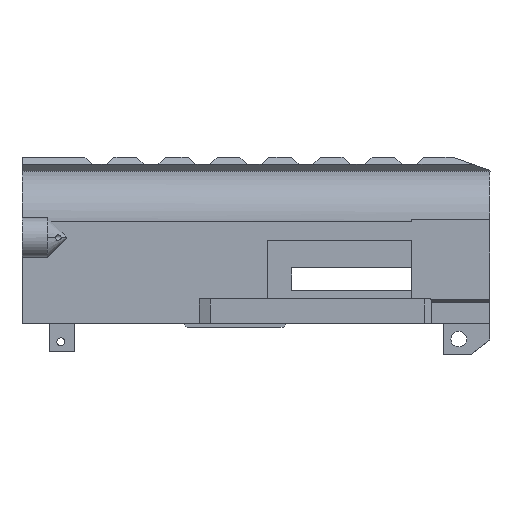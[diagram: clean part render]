
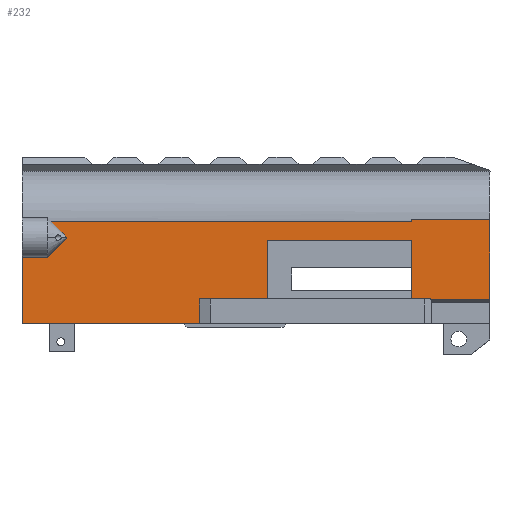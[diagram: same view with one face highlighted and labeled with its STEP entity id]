
A CAD part, top view. The second image highlights one B-rep face of the part: STEP entity #232.
In plain terms, the highlighted planar face has unit normal (0, 0, 1).
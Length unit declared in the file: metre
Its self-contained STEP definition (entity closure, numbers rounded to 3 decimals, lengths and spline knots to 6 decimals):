
#232=ADVANCED_FACE('5:5640',(#699),#700,.T.);
#699=FACE_OUTER_BOUND('',#1312,.T.);
#700=PLANE('',#1313);
#1312=EDGE_LOOP('',(#3033,#3034,#3035,#3036,#3037,#3038,#3039,#3040,#3041,#3042,#3043,#3044,#3045,#3046,#3047,#3048,#3049,#3050));
#1313=AXIS2_PLACEMENT_3D('',#3051,#3052,#3053);
#3033=ORIENTED_EDGE('',*,*,#4156,.T.);
#3034=ORIENTED_EDGE('',*,*,#4449,.T.);
#3035=ORIENTED_EDGE('',*,*,#4154,.F.);
#3036=ORIENTED_EDGE('',*,*,#4429,.F.);
#3037=ORIENTED_EDGE('',*,*,#4450,.T.);
#3038=ORIENTED_EDGE('',*,*,#4401,.F.);
#3039=ORIENTED_EDGE('',*,*,#4002,.F.);
#3040=ORIENTED_EDGE('',*,*,#4430,.F.);
#3041=ORIENTED_EDGE('',*,*,#4140,.T.);
#3042=ORIENTED_EDGE('',*,*,#4122,.F.);
#3043=ORIENTED_EDGE('',*,*,#4451,.T.);
#3044=ORIENTED_EDGE('',*,*,#4118,.F.);
#3045=ORIENTED_EDGE('',*,*,#4117,.F.);
#3046=ORIENTED_EDGE('',*,*,#4116,.T.);
#3047=ORIENTED_EDGE('',*,*,#3915,.T.);
#3048=ORIENTED_EDGE('',*,*,#4452,.T.);
#3049=ORIENTED_EDGE('',*,*,#4399,.F.);
#3050=ORIENTED_EDGE('',*,*,#4395,.T.);
#3051=CARTESIAN_POINT('',(-0.001544,-0.005067,0.0201));
#3052=DIRECTION('',(0.0,0.,1.0));
#3053=DIRECTION('',(-1.0,0.0,0.0));
#3915=EDGE_CURVE('5:7011',#4785,#4783,#4786,.T.);
#4002=EDGE_CURVE('5:6045',#4935,#4937,#4938,.T.);
#4116=EDGE_CURVE('5:7008',#5139,#4785,#5140,.T.);
#4117=EDGE_CURVE('5:7005',#5139,#5141,#5142,.T.);
#4118=EDGE_CURVE('5:7002',#5141,#5143,#5144,.T.);
#4122=EDGE_CURVE('5:6999',#5149,#5151,#5152,.T.);
#4140=EDGE_CURVE('5:6996',#5178,#5151,#5179,.T.);
#4154=EDGE_CURVE('5:6984',#5200,#5198,#5202,.T.);
#4156=EDGE_CURVE('5:6981',#5206,#5204,#5207,.T.);
#4395=EDGE_CURVE('5:7017',#5586,#5206,#5587,.T.);
#4399=EDGE_CURVE('5:7014',#5586,#5592,#5593,.T.);
#4401=EDGE_CURVE('5:6990',#4937,#5595,#5596,.T.);
#4429=EDGE_CURVE('5:6987',#5628,#5200,#5630,.T.);
#4430=EDGE_CURVE('5:6993',#5178,#4935,#5631,.T.);
#4449=EDGE_CURVE('5:6291',#5204,#5198,#5657,.T.);
#4450=EDGE_CURVE('5:6492',#5628,#5595,#5658,.T.);
#4451=EDGE_CURVE('5:6204',#5149,#5143,#5659,.T.);
#4452=EDGE_CURVE('5:6504',#4783,#5592,#5660,.T.);
#4783=VERTEX_POINT('',#6201);
#4785=VERTEX_POINT('',#6203);
#4786=LINE('',#6204,#6205);
#4935=VERTEX_POINT('',#6596);
#4937=VERTEX_POINT('',#6599);
#4938=LINE('',#6600,#6601);
#5139=VERTEX_POINT('',#6893);
#5140=LINE('',#6894,#6895);
#5141=VERTEX_POINT('',#6896);
#5142=CIRCLE('',#6897,0.0201);
#5143=VERTEX_POINT('',#6898);
#5144=LINE('',#6899,#6900);
#5149=VERTEX_POINT('',#6906);
#5151=VERTEX_POINT('',#6908);
#5152=LINE('',#6909,#6910);
#5178=VERTEX_POINT('',#6954);
#5179=LINE('',#6955,#6956);
#5198=VERTEX_POINT('',#6986);
#5200=VERTEX_POINT('',#6989);
#5202=LINE('',#6992,#6993);
#5204=VERTEX_POINT('',#6995);
#5206=VERTEX_POINT('',#6998);
#5207=LINE('',#6999,#7000);
#5586=VERTEX_POINT('',#7599);
#5587=LINE('',#7600,#7601);
#5592=VERTEX_POINT('',#7621);
#5593=LINE('',#7622,#7623);
#5595=VERTEX_POINT('',#7625);
#5596=LINE('',#7626,#7627);
#5628=VERTEX_POINT('',#7679);
#5630=LINE('',#7682,#7683);
#5631=LINE('',#7684,#7685);
#5657=LINE('',#7751,#7752);
#5658=LINE('',#7753,#7754);
#5659=LINE('',#7755,#7756);
#5660=LINE('',#7757,#7758);
#6201=CARTESIAN_POINT('',(-0.159682,0.0415,0.0201));
#6203=CARTESIAN_POINT('',(-0.166095,0.047913,0.0201));
#6204=CARTESIAN_POINT('',(-0.159482,0.0413,0.0201));
#6205=VECTOR('',#8150,0.009069);
#6596=CARTESIAN_POINT('',(-0.019032,0.016363,0.0201));
#6599=CARTESIAN_POINT('',(-0.019032,0.039948,0.0201));
#6600=CARTESIAN_POINT('',(-0.019032,0.017441,0.0201));
#6601=VECTOR('',#8292,0.023586);
#6893=CARTESIAN_POINT('',(-0.01905,0.047913,0.0201));
#6894=CARTESIAN_POINT('',(-0.01905,0.047913,0.0201));
#6895=VECTOR('',#8450,0.147045);
#6896=CARTESIAN_POINT('',(-0.01905,0.048502,0.020096));
#6897=AXIS2_PLACEMENT_3D('',#8451,#8452,#8453);
#6898=CARTESIAN_POINT('',(0.0127,0.048502,0.020096));
#6899=CARTESIAN_POINT('',(-0.19405,0.048472,0.020092));
#6900=VECTOR('',#8454,0.03175);
#6906=CARTESIAN_POINT('',(0.0127,0.016229,0.0201));
#6908=CARTESIAN_POINT('',(-0.011605,0.016229,0.0201));
#6909=CARTESIAN_POINT('',(-0.01905,0.016229,0.0201));
#6910=VECTOR('',#8462,0.024305);
#6954=CARTESIAN_POINT('',(-0.011605,0.016363,0.0201));
#6955=CARTESIAN_POINT('',(-0.011605,0.005648,0.0201));
#6956=VECTOR('',#8490,0.000134);
#6986=CARTESIAN_POINT('',(-0.105565,0.006363,0.0201));
#6989=CARTESIAN_POINT('',(-0.105565,0.016363,0.0201));
#6992=CARTESIAN_POINT('',(-0.105565,0.000648,0.0201));
#6993=VECTOR('',#8504,0.000134);
#6995=CARTESIAN_POINT('',(-0.177682,0.006363,0.0201));
#6998=CARTESIAN_POINT('',(-0.177682,0.0333,0.0201));
#6999=CARTESIAN_POINT('',(-0.177682,0.012778,0.0201));
#7000=VECTOR('',#8506,0.001627);
#7599=CARTESIAN_POINT('',(-0.167482,0.0333,0.0201));
#7600=CARTESIAN_POINT('',(-0.167682,0.0333,0.0201));
#7601=VECTOR('',#8808,0.0102);
#7621=CARTESIAN_POINT('',(-0.159682,0.0411,0.0201));
#7622=CARTESIAN_POINT('',(-0.159482,0.0413,0.0201));
#7623=VECTOR('',#8812,0.011031);
#7625=CARTESIAN_POINT('',(-0.078,0.039948,0.0201));
#7626=CARTESIAN_POINT('',(-0.039772,0.039948,0.0201));
#7627=VECTOR('',#8816,0.000018);
#7679=CARTESIAN_POINT('',(-0.078,0.016363,0.0201));
#7682=CARTESIAN_POINT('',(-0.053554,0.016363,0.0201));
#7683=VECTOR('',#8868,0.027565);
#7684=CARTESIAN_POINT('',(-0.053554,0.016363,0.0201));
#7685=VECTOR('',#8869,0.007427);
#7751=CARTESIAN_POINT('',(-0.0435,0.006363,0.0201));
#7752=VECTOR('',#8899,0.072117);
#7753=CARTESIAN_POINT('',(-0.078,0.016363,0.0201));
#7754=VECTOR('',#8900,0.007988);
#7755=CARTESIAN_POINT('',(0.0127,0.004007,0.0201));
#7756=VECTOR('',#8901,0.032303);
#7757=CARTESIAN_POINT('',(-0.159682,0.047463,0.0201));
#7758=VECTOR('',#8902,0.0004);
#8150=DIRECTION('',(0.707,-0.707,0.0));
#8292=DIRECTION('',(0.0,1.0,0.));
#8450=DIRECTION('',(-1.0,0.0,0.0));
#8451=CARTESIAN_POINT('',(-0.01905,0.047913,0.));
#8452=DIRECTION('',(-1.0,0.0,0.0));
#8453=DIRECTION('',(0.0,-1.0,0.0));
#8454=DIRECTION('',(1.0,0.0,0.0));
#8462=DIRECTION('',(-1.0,0.0,0.0));
#8490=DIRECTION('',(0.,-1.0,0.));
#8504=DIRECTION('',(0.0,-1.0,0.));
#8506=DIRECTION('',(0.0,-1.0,0.));
#8808=DIRECTION('',(-1.0,0.0,0.0));
#8812=DIRECTION('',(0.707,0.707,0.0));
#8816=DIRECTION('',(-1.0,0.0,0.0));
#8868=DIRECTION('',(-1.0,0.0,0.0));
#8869=DIRECTION('',(-1.0,0.0,0.0));
#8899=DIRECTION('',(1.0,0.0,0.0));
#8900=DIRECTION('',(0.0,1.0,0.0));
#8901=DIRECTION('',(0.0,1.0,0.));
#8902=DIRECTION('',(0.0,-1.0,0.0));
